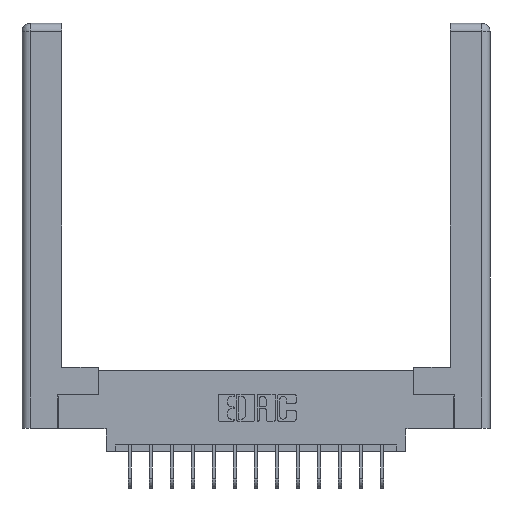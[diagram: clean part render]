
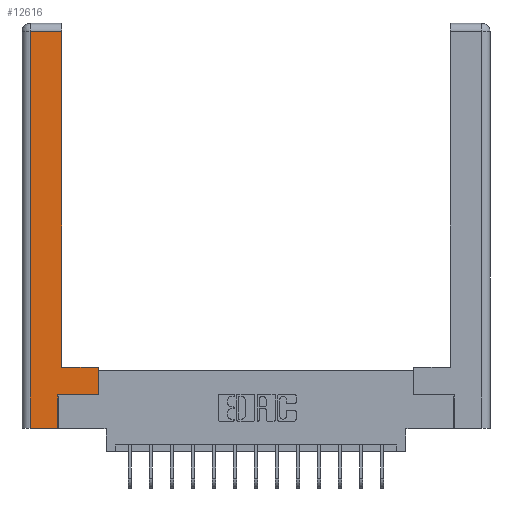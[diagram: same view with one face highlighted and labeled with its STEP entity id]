
A CAD part, top view. The second image highlights one B-rep face of the part: STEP entity #12616.
In plain terms, the highlighted planar face has unit normal (0, 0, 1).
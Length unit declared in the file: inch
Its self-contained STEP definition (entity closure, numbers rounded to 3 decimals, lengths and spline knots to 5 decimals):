
#166 = EDGE_CURVE ( 'NONE', #2525, #17213, #11765, .T. ) ;
#265 = CARTESIAN_POINT ( 'NONE',  ( 0.0615, 0., 0. ) ) ;
#443 = EDGE_CURVE ( 'NONE', #12465, #12872, #15079, .T. ) ;
#757 = EDGE_LOOP ( 'NONE', ( #5593, #1884, #5609, #9375, #17176, #15887, #1235, #16213 ) ) ;
#1235 = ORIENTED_EDGE ( 'NONE', *, *, #3582, .T. ) ;
#1884 = ORIENTED_EDGE ( 'NONE', *, *, #18145, .T. ) ;
#2525 = VERTEX_POINT ( 'NONE', #3651 ) ;
#2814 = PLANE ( 'NONE',  #15678 ) ;
#3582 = EDGE_CURVE ( 'NONE', #9114, #2525, #13622, .T. ) ;
#3651 = CARTESIAN_POINT ( 'NONE',  ( 0.565, 0.45, 0. ) ) ;
#3756 = VECTOR ( 'NONE', #11471, 39.37008 ) ;
#4040 = CARTESIAN_POINT ( 'NONE',  ( 0.265, 0., 0. ) ) ;
#4088 = CARTESIAN_POINT ( 'NONE',  ( 0.565, 0.245, 0. ) ) ;
#4724 = VECTOR ( 'NONE', #16182, 39.37008 ) ;
#5047 = LINE ( 'NONE', #16113, #10179 ) ;
#5593 = ORIENTED_EDGE ( 'NONE', *, *, #14187, .T. ) ;
#5609 = ORIENTED_EDGE ( 'NONE', *, *, #443, .T. ) ;
#5671 = CARTESIAN_POINT ( 'NONE',  ( 0.565, 0.245, 0. ) ) ;
#5770 = DIRECTION ( 'NONE',  ( 0., -1., 0. ) ) ;
#5938 = VECTOR ( 'NONE', #12649, 39.37008 ) ;
#6178 = VERTEX_POINT ( 'NONE', #10542 ) ;
#6462 = EDGE_CURVE ( 'NONE', #17639, #9114, #13472, .T. ) ;
#7341 = EDGE_CURVE ( 'NONE', #12872, #6178, #17244, .T. ) ;
#7547 = VECTOR ( 'NONE', #5770, 39.37008 ) ;
#7947 = CARTESIAN_POINT ( 'NONE',  ( 0.295, 3., 0. ) ) ;
#8232 = DIRECTION ( 'NONE',  ( 1., 0., 0. ) ) ;
#8498 = CARTESIAN_POINT ( 'NONE',  ( 0., 0., 0. ) ) ;
#8794 = CARTESIAN_POINT ( 'NONE',  ( 0.565, 0.45, 0. ) ) ;
#8812 = CARTESIAN_POINT ( 'NONE',  ( 0.295, 0.45, 0. ) ) ;
#8909 = DIRECTION ( 'NONE',  ( 0., 1., 0. ) ) ;
#8984 = VECTOR ( 'NONE', #18305, 39.37008 ) ;
#9114 = VERTEX_POINT ( 'NONE', #5671 ) ;
#9375 = ORIENTED_EDGE ( 'NONE', *, *, #7341, .T. ) ;
#9958 = VECTOR ( 'NONE', #8909, 39.37008 ) ;
#10179 = VECTOR ( 'NONE', #15878, 39.37008 ) ;
#10315 = CARTESIAN_POINT ( 'NONE',  ( 0.265, 0.245, 0. ) ) ;
#10542 = CARTESIAN_POINT ( 'NONE',  ( 0.265, 0., 0. ) ) ;
#10544 = CARTESIAN_POINT ( 'NONE',  ( 0.0615, 0., 0. ) ) ;
#10666 = EDGE_CURVE ( 'NONE', #6178, #17639, #13968, .T. ) ;
#11018 = CARTESIAN_POINT ( 'NONE',  ( 0.295, 2.94, 0. ) ) ;
#11061 = CARTESIAN_POINT ( 'NONE',  ( 0.265, 0.245, 0. ) ) ;
#11471 = DIRECTION ( 'NONE',  ( -1., 0., 0. ) ) ;
#11762 = CARTESIAN_POINT ( 'NONE',  ( 0.0615, 2.94, 0. ) ) ;
#11765 = LINE ( 'NONE', #8812, #3756 ) ;
#12465 = VERTEX_POINT ( 'NONE', #11762 ) ;
#12616 = ADVANCED_FACE ( 'NONE', ( #15857 ), #2814, .F. ) ;
#12649 = DIRECTION ( 'NONE',  ( 1., 0., 0. ) ) ;
#12872 = VERTEX_POINT ( 'NONE', #10544 ) ;
#13161 = VERTEX_POINT ( 'NONE', #11018 ) ;
#13472 = LINE ( 'NONE', #4088, #5938 ) ;
#13622 = LINE ( 'NONE', #8794, #4724 ) ;
#13968 = LINE ( 'NONE', #10315, #9958 ) ;
#14109 = DIRECTION ( 'NONE',  ( 0., 0., -1. ) ) ;
#14120 = VECTOR ( 'NONE', #8232, 39.37008 ) ;
#14187 = EDGE_CURVE ( 'NONE', #17213, #13161, #16503, .T. ) ;
#14225 = CARTESIAN_POINT ( 'NONE',  ( 0.295, 0.45, 0. ) ) ;
#15079 = LINE ( 'NONE', #265, #7547 ) ;
#15342 = DIRECTION ( 'NONE',  ( -1., 0., 0. ) ) ;
#15678 = AXIS2_PLACEMENT_3D ( 'NONE', #8498, #14109, #15342 ) ;
#15857 = FACE_OUTER_BOUND ( 'NONE', #757, .T. ) ;
#15878 = DIRECTION ( 'NONE',  ( -1., 0., 0. ) ) ;
#15887 = ORIENTED_EDGE ( 'NONE', *, *, #6462, .T. ) ;
#16113 = CARTESIAN_POINT ( 'NONE',  ( 0.0615, 2.94, 0. ) ) ;
#16182 = DIRECTION ( 'NONE',  ( 0., 1., 0. ) ) ;
#16213 = ORIENTED_EDGE ( 'NONE', *, *, #166, .T. ) ;
#16503 = LINE ( 'NONE', #7947, #8984 ) ;
#17176 = ORIENTED_EDGE ( 'NONE', *, *, #10666, .T. ) ;
#17213 = VERTEX_POINT ( 'NONE', #14225 ) ;
#17244 = LINE ( 'NONE', #4040, #14120 ) ;
#17639 = VERTEX_POINT ( 'NONE', #11061 ) ;
#18145 = EDGE_CURVE ( 'NONE', #13161, #12465, #5047, .T. ) ;
#18305 = DIRECTION ( 'NONE',  ( 0., 1., 0. ) ) ;
